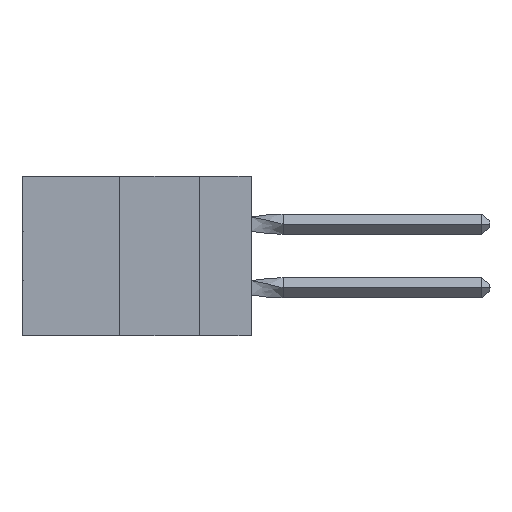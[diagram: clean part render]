
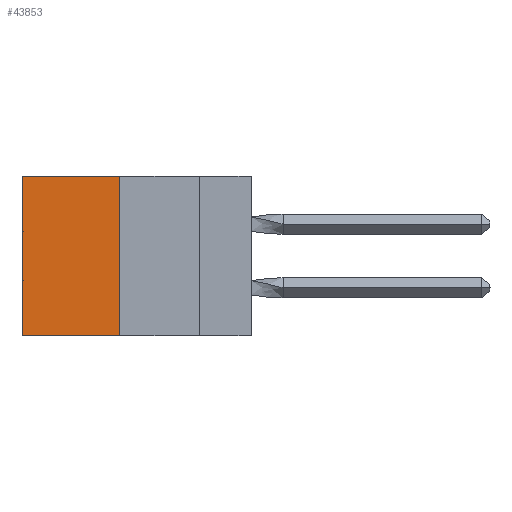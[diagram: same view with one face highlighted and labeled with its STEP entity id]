
A CAD part, left-side view. The second image highlights one B-rep face of the part: STEP entity #43853.
In plain terms, the highlighted planar face has unit normal (-1, 0, 0).
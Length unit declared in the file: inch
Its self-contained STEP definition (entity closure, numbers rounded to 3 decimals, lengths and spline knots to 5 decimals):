
#118 = EDGE_CURVE ( 'NONE', #37670, #12792, #19746, .T. ) ;
#1168 = CARTESIAN_POINT ( 'NONE',  ( 0.305, 0.413, -0.5 ) ) ;
#1321 = ORIENTED_EDGE ( 'NONE', *, *, #30253, .T. ) ;
#2299 = VECTOR ( 'NONE', #19869, 39.37008 ) ;
#6547 = CARTESIAN_POINT ( 'NONE',  ( 0.305, 0.413, -0.5 ) ) ;
#6726 = VECTOR ( 'NONE', #44747, 39.37008 ) ;
#7130 = LINE ( 'NONE', #9814, #2299 ) ;
#7430 = DIRECTION ( 'NONE',  ( 0., 1., 0. ) ) ;
#9336 = CARTESIAN_POINT ( 'NONE',  ( 0.305, 0.72, 0. ) ) ;
#9814 = CARTESIAN_POINT ( 'NONE',  ( 0.305, 0.72, -0.5 ) ) ;
#11650 = ORIENTED_EDGE ( 'NONE', *, *, #118, .F. ) ;
#12792 = VERTEX_POINT ( 'NONE', #1168 ) ;
#12848 = DIRECTION ( 'NONE',  ( 1., 0., 0. ) ) ;
#14590 = VECTOR ( 'NONE', #22850, 39.37008 ) ;
#15467 = EDGE_CURVE ( 'NONE', #12792, #40618, #36890, .T. ) ;
#19746 = LINE ( 'NONE', #6547, #6726 ) ;
#19869 = DIRECTION ( 'NONE',  ( 0., 0., -1. ) ) ;
#20155 = PLANE ( 'NONE',  #42493 ) ;
#22850 = DIRECTION ( 'NONE',  ( 0., 1., 0. ) ) ;
#23132 = EDGE_LOOP ( 'NONE', ( #41115, #43108, #11650, #1321 ) ) ;
#28080 = CARTESIAN_POINT ( 'NONE',  ( 0.305, 0.413, 0. ) ) ;
#28954 = CARTESIAN_POINT ( 'NONE',  ( 0.305, 0.413, -0.5 ) ) ;
#29474 = CARTESIAN_POINT ( 'NONE',  ( 0.305, 0.72, -0.5 ) ) ;
#30253 = EDGE_CURVE ( 'NONE', #37670, #31140, #41423, .T. ) ;
#31140 = VERTEX_POINT ( 'NONE', #9336 ) ;
#34222 = CARTESIAN_POINT ( 'NONE',  ( 0.305, 0.413, 0. ) ) ;
#35466 = VECTOR ( 'NONE', #7430, 39.37008 ) ;
#36890 = LINE ( 'NONE', #28954, #14590 ) ;
#37670 = VERTEX_POINT ( 'NONE', #34222 ) ;
#38918 = EDGE_CURVE ( 'NONE', #31140, #40618, #7130, .T. ) ;
#40519 = DIRECTION ( 'NONE',  ( 0., 0., -1. ) ) ;
#40618 = VERTEX_POINT ( 'NONE', #29474 ) ;
#41115 = ORIENTED_EDGE ( 'NONE', *, *, #38918, .T. ) ;
#41423 = LINE ( 'NONE', #28080, #35466 ) ;
#42493 = AXIS2_PLACEMENT_3D ( 'NONE', #44271, #12848, #40519 ) ;
#43108 = ORIENTED_EDGE ( 'NONE', *, *, #15467, .F. ) ;
#43853 = ADVANCED_FACE ( 'NONE', ( #44576 ), #20155, .F. ) ;
#44271 = CARTESIAN_POINT ( 'NONE',  ( 0.305, 0.413, -0.5 ) ) ;
#44576 = FACE_OUTER_BOUND ( 'NONE', #23132, .T. ) ;
#44747 = DIRECTION ( 'NONE',  ( 0., 0., -1. ) ) ;
